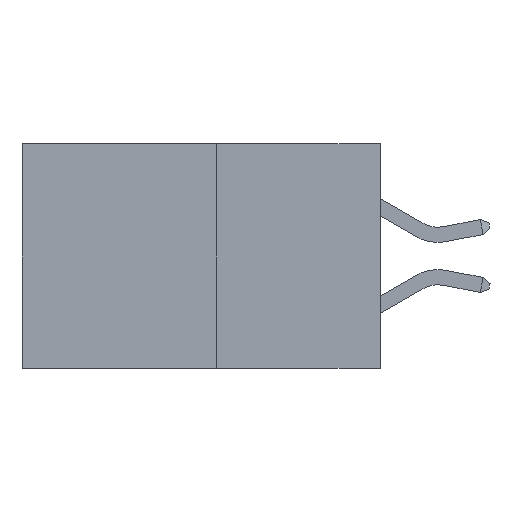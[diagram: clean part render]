
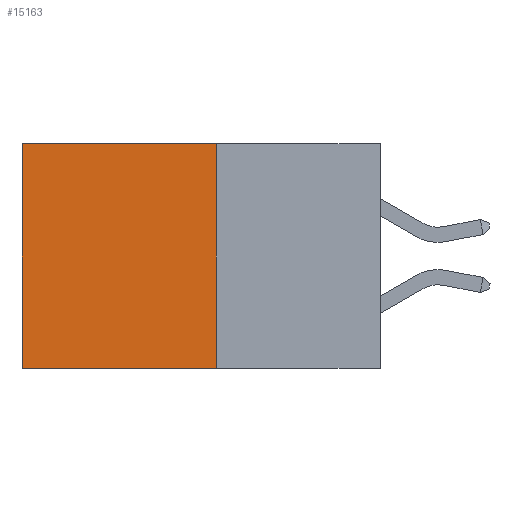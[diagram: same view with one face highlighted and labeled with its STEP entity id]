
A CAD part, left-side view. The second image highlights one B-rep face of the part: STEP entity #15163.
In plain terms, the highlighted planar face has unit normal (-1, 0, 0).
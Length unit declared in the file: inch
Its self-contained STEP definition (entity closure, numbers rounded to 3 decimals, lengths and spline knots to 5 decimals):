
#1755 = CARTESIAN_POINT ( 'NONE',  ( 0.277, 0.59, -0.37 ) ) ;
#2277 = CARTESIAN_POINT ( 'NONE',  ( 0.277, 0.59, 0. ) ) ;
#2351 = DIRECTION ( 'NONE',  ( 0., 0., -1. ) ) ;
#2551 = VECTOR ( 'NONE', #15526, 39.37008 ) ;
#3256 = CARTESIAN_POINT ( 'NONE',  ( 0.277, 0.27, -0.37 ) ) ;
#3562 = DIRECTION ( 'NONE',  ( 0., 1., 0. ) ) ;
#3606 = VERTEX_POINT ( 'NONE', #2277 ) ;
#4172 = VERTEX_POINT ( 'NONE', #1755 ) ;
#4259 = CARTESIAN_POINT ( 'NONE',  ( 0.277, 0.27, -0.37 ) ) ;
#4466 = CARTESIAN_POINT ( 'NONE',  ( 0.277, 0.27, -0.37 ) ) ;
#5311 = EDGE_LOOP ( 'NONE', ( #14894, #20258, #9015, #12470 ) ) ;
#6562 = VECTOR ( 'NONE', #18242, 39.37008 ) ;
#7439 = CARTESIAN_POINT ( 'NONE',  ( 0.277, 0.27, 0. ) ) ;
#7916 = PLANE ( 'NONE',  #17536 ) ;
#8099 = VERTEX_POINT ( 'NONE', #7439 ) ;
#9015 = ORIENTED_EDGE ( 'NONE', *, *, #13367, .F. ) ;
#9715 = VERTEX_POINT ( 'NONE', #4466 ) ;
#10083 = EDGE_CURVE ( 'NONE', #8099, #3606, #17364, .T. ) ;
#11550 = LINE ( 'NONE', #3256, #6562 ) ;
#11689 = CARTESIAN_POINT ( 'NONE',  ( 0.277, 0.27, -0.37 ) ) ;
#12470 = ORIENTED_EDGE ( 'NONE', *, *, #10083, .T. ) ;
#12890 = CARTESIAN_POINT ( 'NONE',  ( 0.277, 0.27, 0. ) ) ;
#13367 = EDGE_CURVE ( 'NONE', #8099, #9715, #22755, .T. ) ;
#13565 = DIRECTION ( 'NONE',  ( 1., 0., 0. ) ) ;
#13611 = CARTESIAN_POINT ( 'NONE',  ( 0.277, 0.59, -0.37 ) ) ;
#14894 = ORIENTED_EDGE ( 'NONE', *, *, #15890, .T. ) ;
#15163 = ADVANCED_FACE ( 'NONE', ( #17829 ), #7916, .F. ) ;
#15526 = DIRECTION ( 'NONE',  ( 0., 0., -1. ) ) ;
#15890 = EDGE_CURVE ( 'NONE', #3606, #4172, #21874, .T. ) ;
#17364 = LINE ( 'NONE', #12890, #21735 ) ;
#17463 = EDGE_CURVE ( 'NONE', #9715, #4172, #11550, .T. ) ;
#17536 = AXIS2_PLACEMENT_3D ( 'NONE', #11689, #13565, #2351 ) ;
#17810 = VECTOR ( 'NONE', #21119, 39.37008 ) ;
#17829 = FACE_OUTER_BOUND ( 'NONE', #5311, .T. ) ;
#18242 = DIRECTION ( 'NONE',  ( 0., 1., 0. ) ) ;
#20258 = ORIENTED_EDGE ( 'NONE', *, *, #17463, .F. ) ;
#21119 = DIRECTION ( 'NONE',  ( 0., 0., -1. ) ) ;
#21735 = VECTOR ( 'NONE', #3562, 39.37008 ) ;
#21874 = LINE ( 'NONE', #13611, #2551 ) ;
#22755 = LINE ( 'NONE', #4259, #17810 ) ;
